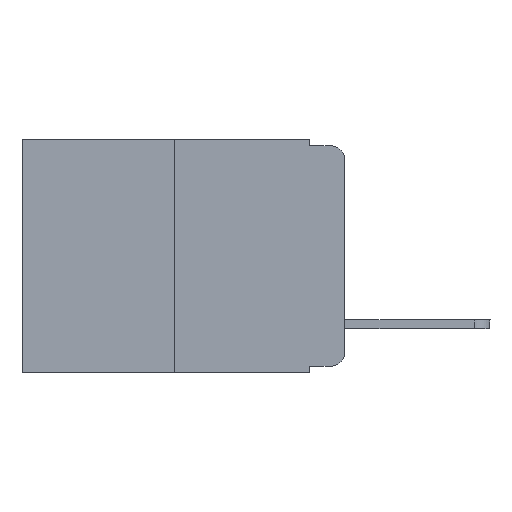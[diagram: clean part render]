
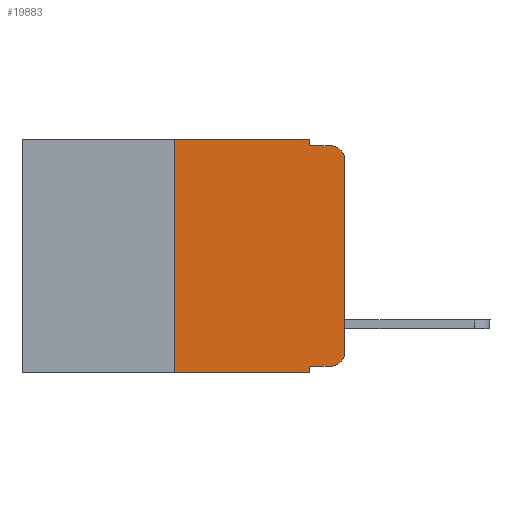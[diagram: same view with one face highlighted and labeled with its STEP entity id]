
A CAD part, left-side view. The second image highlights one B-rep face of the part: STEP entity #19883.
In plain terms, the highlighted planar face has unit normal (-1, 0, 0).
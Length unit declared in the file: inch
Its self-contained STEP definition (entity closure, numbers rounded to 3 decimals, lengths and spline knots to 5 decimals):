
#5 = CARTESIAN_POINT ( 'NONE',  ( 0., 0.051, 0. ) ) ;
#236 = DIRECTION ( 'NONE',  ( 0., 0., 1. ) ) ;
#1436 = ORIENTED_EDGE ( 'NONE', *, *, #10637, .T. ) ;
#1455 = LINE ( 'NONE', #5168, #5664 ) ;
#1527 = CARTESIAN_POINT ( 'NONE',  ( 0., 0., -0.03 ) ) ;
#1763 = ORIENTED_EDGE ( 'NONE', *, *, #18836, .F. ) ;
#2159 = AXIS2_PLACEMENT_3D ( 'NONE', #20263, #9997, #11988 ) ;
#2326 = AXIS2_PLACEMENT_3D ( 'NONE', #2818, #19516, #3036 ) ;
#2388 = DIRECTION ( 'NONE',  ( 0., -1., 0. ) ) ;
#2454 = CARTESIAN_POINT ( 'NONE',  ( 0., 0.473, 0. ) ) ;
#2818 = CARTESIAN_POINT ( 'NONE',  ( 0., 0.02, -0.03 ) ) ;
#3036 = DIRECTION ( 'NONE',  ( 0., 0., -1. ) ) ;
#3107 = CARTESIAN_POINT ( 'NONE',  ( 0., 0.051, -0.343 ) ) ;
#3221 = VERTEX_POINT ( 'NONE', #20262 ) ;
#3226 = EDGE_CURVE ( 'NONE', #19877, #4805, #1455, .T. ) ;
#3275 = DIRECTION ( 'NONE',  ( 0., 0., -1. ) ) ;
#3303 = ORIENTED_EDGE ( 'NONE', *, *, #3782, .T. ) ;
#3493 = EDGE_CURVE ( 'NONE', #21111, #4405, #12212, .T. ) ;
#3583 = VECTOR ( 'NONE', #236, 39.37008 ) ;
#3723 = ORIENTED_EDGE ( 'NONE', *, *, #5897, .F. ) ;
#3782 = EDGE_CURVE ( 'NONE', #18201, #11864, #16870, .T. ) ;
#3974 = CARTESIAN_POINT ( 'NONE',  ( 0., 0.473, 0. ) ) ;
#4405 = VERTEX_POINT ( 'NONE', #20029 ) ;
#4422 = CARTESIAN_POINT ( 'NONE',  ( 0., 0.051, 0. ) ) ;
#4805 = VERTEX_POINT ( 'NONE', #19097 ) ;
#5168 = CARTESIAN_POINT ( 'NONE',  ( 0., 0.051, -0.333 ) ) ;
#5186 = VECTOR ( 'NONE', #12279, 39.37008 ) ;
#5276 = VECTOR ( 'NONE', #2388, 39.37008 ) ;
#5664 = VECTOR ( 'NONE', #10988, 39.37008 ) ;
#5666 = EDGE_CURVE ( 'NONE', #4805, #18201, #11241, .T. ) ;
#5897 = EDGE_CURVE ( 'NONE', #19877, #13593, #6245, .T. ) ;
#6149 = CARTESIAN_POINT ( 'NONE',  ( 0., 0.473, -0.343 ) ) ;
#6245 = LINE ( 'NONE', #10570, #5186 ) ;
#6512 = CARTESIAN_POINT ( 'NONE',  ( 0., 0.051, -0.01 ) ) ;
#6658 = VERTEX_POINT ( 'NONE', #4422 ) ;
#6721 = ORIENTED_EDGE ( 'NONE', *, *, #15285, .T. ) ;
#7194 = DIRECTION ( 'NONE',  ( 0., 0., -1. ) ) ;
#7700 = LINE ( 'NONE', #2454, #5276 ) ;
#7739 = EDGE_LOOP ( 'NONE', ( #3303, #6721, #9387, #8362, #1763, #9100, #1436, #3723, #7878, #19938 ) ) ;
#7878 = ORIENTED_EDGE ( 'NONE', *, *, #3226, .T. ) ;
#8360 = EDGE_CURVE ( 'NONE', #6658, #21111, #18684, .T. ) ;
#8362 = ORIENTED_EDGE ( 'NONE', *, *, #8360, .F. ) ;
#8520 = VECTOR ( 'NONE', #8917, 39.37008 ) ;
#8668 = CARTESIAN_POINT ( 'NONE',  ( 0., 0.051, -0.333 ) ) ;
#8869 = VERTEX_POINT ( 'NONE', #21488 ) ;
#8917 = DIRECTION ( 'NONE',  ( 0., 0., 1. ) ) ;
#8934 = LINE ( 'NONE', #6149, #14953 ) ;
#9025 = PLANE ( 'NONE',  #10673 ) ;
#9100 = ORIENTED_EDGE ( 'NONE', *, *, #16224, .F. ) ;
#9387 = ORIENTED_EDGE ( 'NONE', *, *, #3493, .F. ) ;
#9997 = DIRECTION ( 'NONE',  ( -1., 0., 0. ) ) ;
#10090 = DIRECTION ( 'NONE',  ( 0., -1., 0. ) ) ;
#10552 = DIRECTION ( 'NONE',  ( 1., 0., 0. ) ) ;
#10570 = CARTESIAN_POINT ( 'NONE',  ( 0., 0.051, 0. ) ) ;
#10637 = EDGE_CURVE ( 'NONE', #3221, #13593, #8934, .T. ) ;
#10673 = AXIS2_PLACEMENT_3D ( 'NONE', #3974, #10552, #7194 ) ;
#10988 = DIRECTION ( 'NONE',  ( 0., -1., 0. ) ) ;
#11241 = CIRCLE ( 'NONE', #2159, 0.02 ) ;
#11861 = CARTESIAN_POINT ( 'NONE',  ( 0., 0.25, 0. ) ) ;
#11864 = VERTEX_POINT ( 'NONE', #1527 ) ;
#11988 = DIRECTION ( 'NONE',  ( 0., 0., -1. ) ) ;
#12212 = LINE ( 'NONE', #6512, #21631 ) ;
#12279 = DIRECTION ( 'NONE',  ( 0., 0., -1. ) ) ;
#13593 = VERTEX_POINT ( 'NONE', #3107 ) ;
#13819 = CARTESIAN_POINT ( 'NONE',  ( 0., 0.051, -0.01 ) ) ;
#14953 = VECTOR ( 'NONE', #19546, 39.37008 ) ;
#15203 = FACE_OUTER_BOUND ( 'NONE', #7739, .T. ) ;
#15285 = EDGE_CURVE ( 'NONE', #11864, #4405, #20137, .T. ) ;
#15698 = CARTESIAN_POINT ( 'NONE',  ( 0., 0., 0. ) ) ;
#16224 = EDGE_CURVE ( 'NONE', #3221, #8869, #19277, .T. ) ;
#16870 = LINE ( 'NONE', #15698, #8520 ) ;
#17910 = VECTOR ( 'NONE', #3275, 39.37008 ) ;
#18201 = VERTEX_POINT ( 'NONE', #19070 ) ;
#18684 = LINE ( 'NONE', #5, #17910 ) ;
#18836 = EDGE_CURVE ( 'NONE', #8869, #6658, #7700, .T. ) ;
#19070 = CARTESIAN_POINT ( 'NONE',  ( 0., 0., -0.313 ) ) ;
#19097 = CARTESIAN_POINT ( 'NONE',  ( 0., 0.02, -0.333 ) ) ;
#19277 = LINE ( 'NONE', #11861, #3583 ) ;
#19516 = DIRECTION ( 'NONE',  ( -1., 0., 0. ) ) ;
#19546 = DIRECTION ( 'NONE',  ( 0., -1., 0. ) ) ;
#19877 = VERTEX_POINT ( 'NONE', #8668 ) ;
#19883 = ADVANCED_FACE ( 'NONE', ( #15203 ), #9025, .F. ) ;
#19938 = ORIENTED_EDGE ( 'NONE', *, *, #5666, .T. ) ;
#20029 = CARTESIAN_POINT ( 'NONE',  ( 0., 0.02, -0.01 ) ) ;
#20137 = CIRCLE ( 'NONE', #2326, 0.02 ) ;
#20262 = CARTESIAN_POINT ( 'NONE',  ( 0., 0.25, -0.343 ) ) ;
#20263 = CARTESIAN_POINT ( 'NONE',  ( 0., 0.02, -0.313 ) ) ;
#21111 = VERTEX_POINT ( 'NONE', #13819 ) ;
#21488 = CARTESIAN_POINT ( 'NONE',  ( 0., 0.25, 0. ) ) ;
#21631 = VECTOR ( 'NONE', #10090, 39.37008 ) ;
